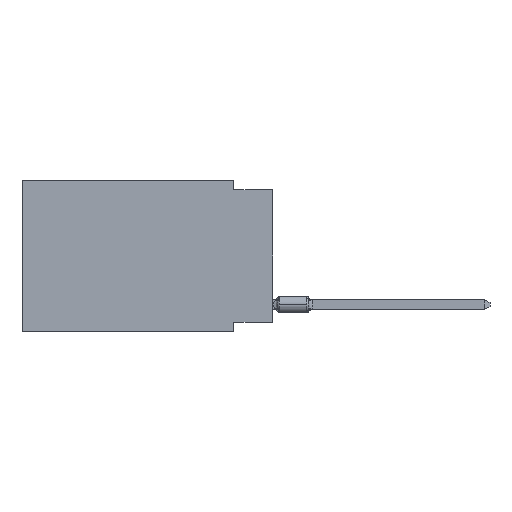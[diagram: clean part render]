
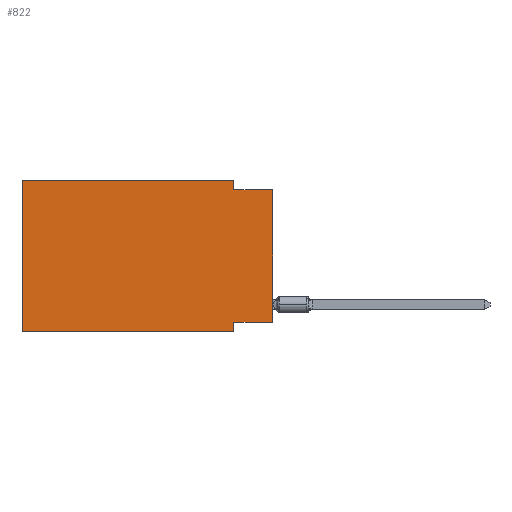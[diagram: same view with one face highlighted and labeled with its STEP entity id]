
A CAD part, left-side view. The second image highlights one B-rep face of the part: STEP entity #822.
In plain terms, the highlighted planar face has unit normal (-1, 0, 0).
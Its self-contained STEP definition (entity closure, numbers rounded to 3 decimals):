
#64 = LINE ( 'NONE', #20786, #7253 ) ;
#745 = CARTESIAN_POINT ( 'NONE',  ( 0., 0., -0.635 ) ) ;
#822 = ADVANCED_FACE ( 'NONE', ( #15354 ), #13877, .F. ) ;
#853 = LINE ( 'NONE', #745, #16619 ) ;
#1021 = VECTOR ( 'NONE', #7076, 1000. ) ;
#1040 = EDGE_CURVE ( 'NONE', #10025, #16110, #20190, .T. ) ;
#1551 = DIRECTION ( 'NONE',  ( 0., 0., -1. ) ) ;
#1599 = VERTEX_POINT ( 'NONE', #12121 ) ;
#2554 = DIRECTION ( 'NONE',  ( 0., -1., 0. ) ) ;
#2856 = LINE ( 'NONE', #3312, #13759 ) ;
#3047 = ORIENTED_EDGE ( 'NONE', *, *, #14677, .T. ) ;
#3292 = CARTESIAN_POINT ( 'NONE',  ( 0., 16.383, 0. ) ) ;
#3312 = CARTESIAN_POINT ( 'NONE',  ( 0., 16.383, 0. ) ) ;
#3563 = DIRECTION ( 'NONE',  ( 0., -1., 0. ) ) ;
#3633 = VERTEX_POINT ( 'NONE', #4825 ) ;
#3955 = LINE ( 'NONE', #19687, #19141 ) ;
#4222 = CARTESIAN_POINT ( 'NONE',  ( 0., 16.383, -9.906 ) ) ;
#4645 = ORIENTED_EDGE ( 'NONE', *, *, #19618, .T. ) ;
#4825 = CARTESIAN_POINT ( 'NONE',  ( 0., 2.54, 0. ) ) ;
#5536 = CARTESIAN_POINT ( 'NONE',  ( 0., 0., -0.635 ) ) ;
#5720 = EDGE_CURVE ( 'NONE', #16277, #19758, #853, .T. ) ;
#6834 = VECTOR ( 'NONE', #15337, 1000. ) ;
#7076 = DIRECTION ( 'NONE',  ( 0., 0., -1. ) ) ;
#7253 = VECTOR ( 'NONE', #3563, 1000. ) ;
#7559 = VECTOR ( 'NONE', #16949, 1000. ) ;
#8328 = ORIENTED_EDGE ( 'NONE', *, *, #21980, .F. ) ;
#8398 = ORIENTED_EDGE ( 'NONE', *, *, #21125, .F. ) ;
#8449 = CARTESIAN_POINT ( 'NONE',  ( 0., 0., -9.271 ) ) ;
#8644 = EDGE_CURVE ( 'NONE', #3633, #16277, #14026, .T. ) ;
#9175 = DIRECTION ( 'NONE',  ( 0., 0., 1. ) ) ;
#9541 = VERTEX_POINT ( 'NONE', #4222 ) ;
#10025 = VERTEX_POINT ( 'NONE', #18327 ) ;
#10732 = CARTESIAN_POINT ( 'NONE',  ( 0., 2.54, -9.906 ) ) ;
#11283 = EDGE_LOOP ( 'NONE', ( #3047, #12145, #15388, #19177, #8398, #4645, #16228, #8328 ) ) ;
#11594 = CARTESIAN_POINT ( 'NONE',  ( 0., 2.54, -9.906 ) ) ;
#11860 = CARTESIAN_POINT ( 'NONE',  ( 0., 16.383, -9.906 ) ) ;
#12016 = DIRECTION ( 'NONE',  ( 0., 0., -1. ) ) ;
#12121 = CARTESIAN_POINT ( 'NONE',  ( 0., 0., -9.271 ) ) ;
#12145 = ORIENTED_EDGE ( 'NONE', *, *, #5720, .F. ) ;
#12226 = CARTESIAN_POINT ( 'NONE',  ( 0., 2.54, 0. ) ) ;
#12231 = AXIS2_PLACEMENT_3D ( 'NONE', #15460, #15684, #1551 ) ;
#13723 = VERTEX_POINT ( 'NONE', #3292 ) ;
#13755 = LINE ( 'NONE', #8449, #6834 ) ;
#13759 = VECTOR ( 'NONE', #16668, 1000. ) ;
#13877 = PLANE ( 'NONE',  #12231 ) ;
#14026 = LINE ( 'NONE', #12226, #18185 ) ;
#14151 = EDGE_CURVE ( 'NONE', #13723, #3633, #64, .T. ) ;
#14441 = CARTESIAN_POINT ( 'NONE',  ( 0., 2.54, -0.635 ) ) ;
#14677 = EDGE_CURVE ( 'NONE', #1599, #19758, #3955, .T. ) ;
#15337 = DIRECTION ( 'NONE',  ( 0., 1., 0. ) ) ;
#15354 = FACE_OUTER_BOUND ( 'NONE', #11283, .T. ) ;
#15388 = ORIENTED_EDGE ( 'NONE', *, *, #8644, .F. ) ;
#15460 = CARTESIAN_POINT ( 'NONE',  ( 0., 16.383, 0. ) ) ;
#15684 = DIRECTION ( 'NONE',  ( 1., 0., 0. ) ) ;
#16110 = VERTEX_POINT ( 'NONE', #10732 ) ;
#16228 = ORIENTED_EDGE ( 'NONE', *, *, #1040, .F. ) ;
#16277 = VERTEX_POINT ( 'NONE', #14441 ) ;
#16498 = LINE ( 'NONE', #11860, #7559 ) ;
#16619 = VECTOR ( 'NONE', #2554, 1000. ) ;
#16668 = DIRECTION ( 'NONE',  ( 0., 0., 1. ) ) ;
#16949 = DIRECTION ( 'NONE',  ( 0., -1., 0. ) ) ;
#18185 = VECTOR ( 'NONE', #12016, 1000. ) ;
#18327 = CARTESIAN_POINT ( 'NONE',  ( 0., 2.54, -9.271 ) ) ;
#19141 = VECTOR ( 'NONE', #9175, 1000. ) ;
#19177 = ORIENTED_EDGE ( 'NONE', *, *, #14151, .F. ) ;
#19618 = EDGE_CURVE ( 'NONE', #9541, #16110, #16498, .T. ) ;
#19687 = CARTESIAN_POINT ( 'NONE',  ( 0., 0., 0. ) ) ;
#19758 = VERTEX_POINT ( 'NONE', #5536 ) ;
#20190 = LINE ( 'NONE', #11594, #1021 ) ;
#20786 = CARTESIAN_POINT ( 'NONE',  ( 0., 16.383, 0. ) ) ;
#21125 = EDGE_CURVE ( 'NONE', #9541, #13723, #2856, .T. ) ;
#21980 = EDGE_CURVE ( 'NONE', #1599, #10025, #13755, .T. ) ;
